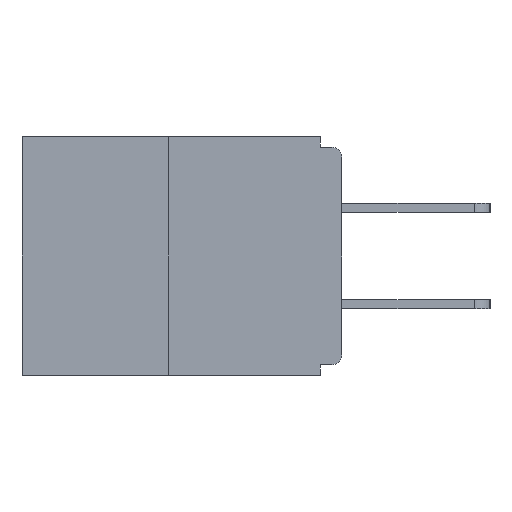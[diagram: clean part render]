
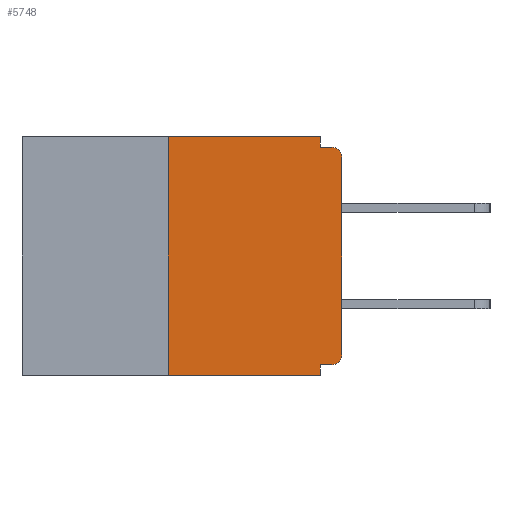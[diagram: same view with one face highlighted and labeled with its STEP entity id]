
A CAD part, left-side view. The second image highlights one B-rep face of the part: STEP entity #5748.
In plain terms, the highlighted planar face has unit normal (-1, 0, 0).
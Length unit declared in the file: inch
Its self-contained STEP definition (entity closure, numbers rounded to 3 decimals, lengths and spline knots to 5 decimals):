
#115 = LINE ( 'NONE', #518, #528 ) ;
#392 = AXIS2_PLACEMENT_3D ( 'NONE', #6335, #17280, #10519 ) ;
#518 = CARTESIAN_POINT ( 'NONE',  ( 0., 0.46, -0.343 ) ) ;
#528 = VECTOR ( 'NONE', #3951, 39.37008 ) ;
#659 = DIRECTION ( 'NONE',  ( -1., 0., 0. ) ) ;
#689 = LINE ( 'NONE', #15573, #1740 ) ;
#887 = VERTEX_POINT ( 'NONE', #12474 ) ;
#1207 = CARTESIAN_POINT ( 'NONE',  ( 0., 0.015, -0.03 ) ) ;
#1235 = LINE ( 'NONE', #13800, #15392 ) ;
#1439 = CARTESIAN_POINT ( 'NONE',  ( 0., 0., 0. ) ) ;
#1740 = VECTOR ( 'NONE', #13494, 39.37008 ) ;
#1925 = AXIS2_PLACEMENT_3D ( 'NONE', #1207, #15798, #3170 ) ;
#1986 = ORIENTED_EDGE ( 'NONE', *, *, #9178, .T. ) ;
#2250 = DIRECTION ( 'NONE',  ( 0., -1., 0. ) ) ;
#2480 = ORIENTED_EDGE ( 'NONE', *, *, #3153, .F. ) ;
#3153 = EDGE_CURVE ( 'NONE', #5086, #11394, #689, .T. ) ;
#3170 = DIRECTION ( 'NONE',  ( 0., 0., -1. ) ) ;
#3252 = CARTESIAN_POINT ( 'NONE',  ( 0., 0.015, -0.328 ) ) ;
#3615 = CARTESIAN_POINT ( 'NONE',  ( 0., 0., -0.328 ) ) ;
#3951 = DIRECTION ( 'NONE',  ( 0., -1., 0. ) ) ;
#4001 = DIRECTION ( 'NONE',  ( 0., 0., 1. ) ) ;
#4045 = LINE ( 'NONE', #1439, #7029 ) ;
#4187 = ORIENTED_EDGE ( 'NONE', *, *, #16754, .F. ) ;
#4192 = VECTOR ( 'NONE', #2250, 39.37008 ) ;
#4501 = VERTEX_POINT ( 'NONE', #13975 ) ;
#4608 = CARTESIAN_POINT ( 'NONE',  ( 0., 0.015, -0.015 ) ) ;
#4838 = EDGE_CURVE ( 'NONE', #11777, #5086, #1235, .T. ) ;
#5086 = VERTEX_POINT ( 'NONE', #12947 ) ;
#5206 = DIRECTION ( 'NONE',  ( 0., 0., 1. ) ) ;
#5748 = ADVANCED_FACE ( 'NONE', ( #8752 ), #7664, .F. ) ;
#6172 = CARTESIAN_POINT ( 'NONE',  ( 0., 0.015, -0.313 ) ) ;
#6200 = CARTESIAN_POINT ( 'NONE',  ( 0., 0.031, 0. ) ) ;
#6335 = CARTESIAN_POINT ( 'NONE',  ( 0., 0.46, 0. ) ) ;
#6345 = DIRECTION ( 'NONE',  ( 0., 0., -1. ) ) ;
#6409 = CIRCLE ( 'NONE', #11474, 0.015 ) ;
#6449 = ORIENTED_EDGE ( 'NONE', *, *, #12849, .F. ) ;
#6511 = CARTESIAN_POINT ( 'NONE',  ( 0., 0.25, 0. ) ) ;
#6888 = VERTEX_POINT ( 'NONE', #12592 ) ;
#7029 = VECTOR ( 'NONE', #4001, 39.37008 ) ;
#7036 = VERTEX_POINT ( 'NONE', #11478 ) ;
#7664 = PLANE ( 'NONE',  #392 ) ;
#7750 = ORIENTED_EDGE ( 'NONE', *, *, #11083, .T. ) ;
#7751 = VECTOR ( 'NONE', #10534, 39.37008 ) ;
#8752 = FACE_OUTER_BOUND ( 'NONE', #11117, .T. ) ;
#8869 = VERTEX_POINT ( 'NONE', #3252 ) ;
#9178 = EDGE_CURVE ( 'NONE', #10803, #7036, #115, .T. ) ;
#9197 = LINE ( 'NONE', #9459, #12446 ) ;
#9459 = CARTESIAN_POINT ( 'NONE',  ( 0., 0.031, -0.343 ) ) ;
#9882 = DIRECTION ( 'NONE',  ( 0., 0., -1. ) ) ;
#10215 = EDGE_CURVE ( 'NONE', #8869, #887, #6409, .T. ) ;
#10519 = DIRECTION ( 'NONE',  ( 0., 0., -1. ) ) ;
#10534 = DIRECTION ( 'NONE',  ( 0., 1., 0. ) ) ;
#10542 = CARTESIAN_POINT ( 'NONE',  ( 0., 0.46, 0. ) ) ;
#10633 = LINE ( 'NONE', #10542, #4192 ) ;
#10803 = VERTEX_POINT ( 'NONE', #14320 ) ;
#11083 = EDGE_CURVE ( 'NONE', #887, #13583, #4045, .T. ) ;
#11102 = VECTOR ( 'NONE', #5206, 39.37008 ) ;
#11117 = EDGE_LOOP ( 'NONE', ( #6449, #17699, #1986, #4187, #12601, #14457, #7750, #15588, #2480, #14218 ) ) ;
#11394 = VERTEX_POINT ( 'NONE', #4608 ) ;
#11474 = AXIS2_PLACEMENT_3D ( 'NONE', #6172, #659, #6345 ) ;
#11478 = CARTESIAN_POINT ( 'NONE',  ( 0., 0.031, -0.343 ) ) ;
#11777 = VERTEX_POINT ( 'NONE', #6200 ) ;
#12383 = EDGE_CURVE ( 'NONE', #10803, #6888, #14653, .T. ) ;
#12446 = VECTOR ( 'NONE', #16472, 39.37008 ) ;
#12474 = CARTESIAN_POINT ( 'NONE',  ( 0., 0., -0.313 ) ) ;
#12592 = CARTESIAN_POINT ( 'NONE',  ( 0., 0.25, 0. ) ) ;
#12601 = ORIENTED_EDGE ( 'NONE', *, *, #17367, .F. ) ;
#12849 = EDGE_CURVE ( 'NONE', #6888, #11777, #10633, .T. ) ;
#12947 = CARTESIAN_POINT ( 'NONE',  ( 0., 0.031, -0.015 ) ) ;
#12973 = EDGE_CURVE ( 'NONE', #13583, #11394, #16626, .T. ) ;
#13494 = DIRECTION ( 'NONE',  ( 0., -1., 0. ) ) ;
#13583 = VERTEX_POINT ( 'NONE', #15387 ) ;
#13800 = CARTESIAN_POINT ( 'NONE',  ( 0., 0.031, 0. ) ) ;
#13975 = CARTESIAN_POINT ( 'NONE',  ( 0., 0.031, -0.328 ) ) ;
#14218 = ORIENTED_EDGE ( 'NONE', *, *, #4838, .F. ) ;
#14320 = CARTESIAN_POINT ( 'NONE',  ( 0., 0.25, -0.343 ) ) ;
#14457 = ORIENTED_EDGE ( 'NONE', *, *, #10215, .T. ) ;
#14653 = LINE ( 'NONE', #6511, #11102 ) ;
#14821 = LINE ( 'NONE', #3615, #7751 ) ;
#15387 = CARTESIAN_POINT ( 'NONE',  ( 0., 0., -0.03 ) ) ;
#15392 = VECTOR ( 'NONE', #9882, 39.37008 ) ;
#15573 = CARTESIAN_POINT ( 'NONE',  ( 0., 0., -0.015 ) ) ;
#15588 = ORIENTED_EDGE ( 'NONE', *, *, #12973, .T. ) ;
#15798 = DIRECTION ( 'NONE',  ( -1., 0., 0. ) ) ;
#16472 = DIRECTION ( 'NONE',  ( 0., 0., -1. ) ) ;
#16626 = CIRCLE ( 'NONE', #1925, 0.015 ) ;
#16754 = EDGE_CURVE ( 'NONE', #4501, #7036, #9197, .T. ) ;
#17280 = DIRECTION ( 'NONE',  ( 1., 0., 0. ) ) ;
#17367 = EDGE_CURVE ( 'NONE', #8869, #4501, #14821, .T. ) ;
#17699 = ORIENTED_EDGE ( 'NONE', *, *, #12383, .F. ) ;
